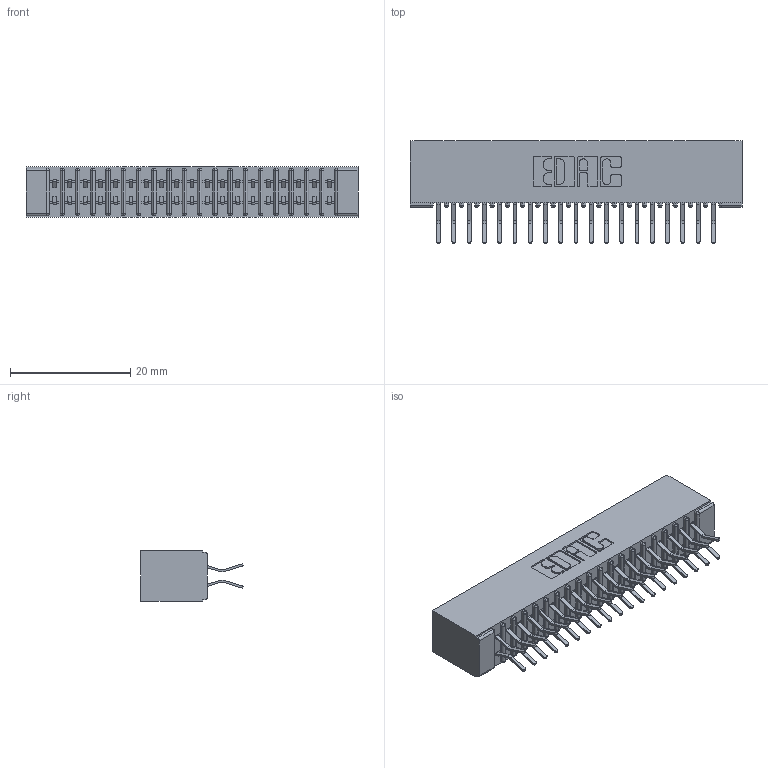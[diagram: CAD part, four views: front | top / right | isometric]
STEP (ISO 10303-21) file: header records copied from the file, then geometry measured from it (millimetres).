
FILE_DESCRIPTION (( 'STEP AP203' ), '1' );
FILE_NAME ('391-038-556-201.STEP', '2018-08-09T00:22:02', ( '' ), ( '' ), 'SwSTEP 2.0', 'SolidWorks 2016', '' );
FILE_SCHEMA (( 'CONFIG_CONTROL_DESIGN' ));
Length unit declared in the file: inch
Products named in the file (3): 341 Part_No Mounting Lugs; 341-292-001_341-292-156; 391-038-556-201
Assembly tree (39 placements, depth 2):
  391-038-556-201
    341 Part_No Mounting Lugs
    341-292-001_341-292-156  x38
Bounding box: 55.24 x 17.07 x 8.38 mm (x, y, z)
Volume: 3294.3 mm3; surface area: 7439.7 mm2
Topology: 39 solids, 39 shells, 2768 faces, 8025 edges, 5206 vertices
Faces by surface type: plane 1584, cylinder 1108, sphere 40, torus 36
Entity records: 25920 total; most frequent: CARTESIAN_POINT 4309, ORIENTED_EDGE 4278, DIRECTION 4201, EDGE_CURVE 2139, VECTOR 1701, LINE 1701, VERTEX_POINT 1358, AXIS2_PLACEMENT_3D 1250
